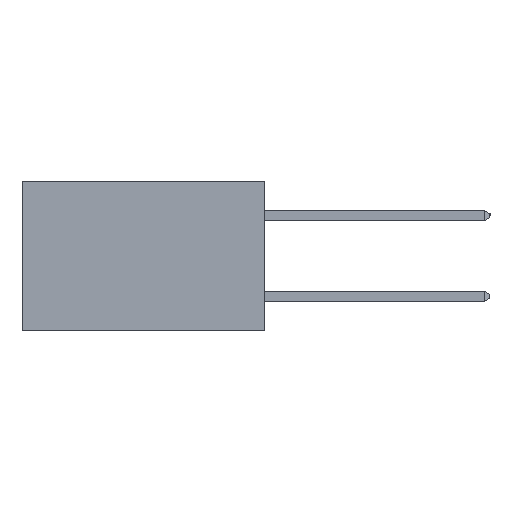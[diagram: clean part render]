
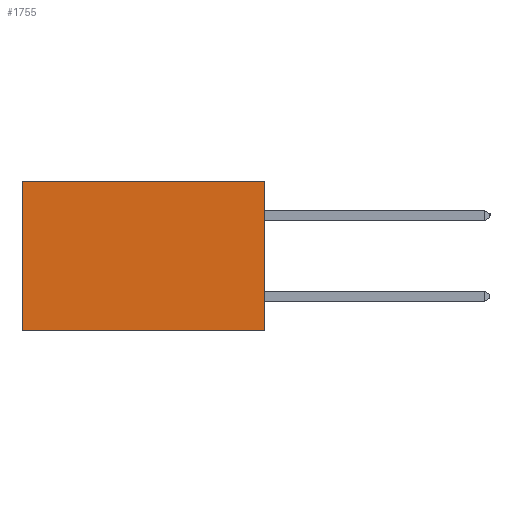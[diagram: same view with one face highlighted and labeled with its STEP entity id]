
A CAD part, left-side view. The second image highlights one B-rep face of the part: STEP entity #1755.
In plain terms, the highlighted planar face has unit normal (-1, 0, 0).
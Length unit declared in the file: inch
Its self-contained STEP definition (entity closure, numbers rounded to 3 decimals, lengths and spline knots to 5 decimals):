
#355 = ORIENTED_EDGE ( 'NONE', *, *, #5531, .T. ) ;
#485 = ORIENTED_EDGE ( 'NONE', *, *, #9100, .F. ) ;
#519 = VERTEX_POINT ( 'NONE', #5094 ) ;
#935 = DIRECTION ( 'NONE',  ( 0., 1., 0. ) ) ;
#1432 = LINE ( 'NONE', #8411, #14731 ) ;
#1681 = LINE ( 'NONE', #14494, #11536 ) ;
#1755 = ADVANCED_FACE ( 'NONE', ( #13725 ), #10812, .F. ) ;
#3118 = ORIENTED_EDGE ( 'NONE', *, *, #9792, .F. ) ;
#3179 = CARTESIAN_POINT ( 'NONE',  ( 0.298, 0., 0. ) ) ;
#3498 = LINE ( 'NONE', #11924, #15955 ) ;
#4749 = EDGE_CURVE ( 'NONE', #14664, #10191, #3498, .T. ) ;
#5094 = CARTESIAN_POINT ( 'NONE',  ( 0.298, 0., -0.37 ) ) ;
#5531 = EDGE_CURVE ( 'NONE', #11937, #14664, #1432, .T. ) ;
#6019 = LINE ( 'NONE', #15826, #15072 ) ;
#7909 = DIRECTION ( 'NONE',  ( 0., 1., 0. ) ) ;
#8411 = CARTESIAN_POINT ( 'NONE',  ( 0.298, 0., 0. ) ) ;
#8684 = DIRECTION ( 'NONE',  ( 0., 0., -1. ) ) ;
#9100 = EDGE_CURVE ( 'NONE', #11937, #519, #1681, .T. ) ;
#9792 = EDGE_CURVE ( 'NONE', #519, #10191, #6019, .T. ) ;
#9852 = CARTESIAN_POINT ( 'NONE',  ( 0.298, 0.6, -0.37 ) ) ;
#10191 = VERTEX_POINT ( 'NONE', #9852 ) ;
#10621 = ORIENTED_EDGE ( 'NONE', *, *, #4749, .T. ) ;
#10795 = CARTESIAN_POINT ( 'NONE',  ( 0.298, 0., 0. ) ) ;
#10812 = PLANE ( 'NONE',  #11677 ) ;
#11536 = VECTOR ( 'NONE', #8684, 39.37008 ) ;
#11677 = AXIS2_PLACEMENT_3D ( 'NONE', #10795, #12424, #12406 ) ;
#11710 = DIRECTION ( 'NONE',  ( 0., 0., -1. ) ) ;
#11924 = CARTESIAN_POINT ( 'NONE',  ( 0.298, 0.6, 0. ) ) ;
#11937 = VERTEX_POINT ( 'NONE', #3179 ) ;
#12406 = DIRECTION ( 'NONE',  ( 0., 0., -1. ) ) ;
#12424 = DIRECTION ( 'NONE',  ( 1., 0., 0. ) ) ;
#13725 = FACE_OUTER_BOUND ( 'NONE', #14390, .T. ) ;
#14390 = EDGE_LOOP ( 'NONE', ( #10621, #3118, #485, #355 ) ) ;
#14494 = CARTESIAN_POINT ( 'NONE',  ( 0.298, 0., 0. ) ) ;
#14664 = VERTEX_POINT ( 'NONE', #15878 ) ;
#14731 = VECTOR ( 'NONE', #7909, 39.37008 ) ;
#15072 = VECTOR ( 'NONE', #935, 39.37008 ) ;
#15826 = CARTESIAN_POINT ( 'NONE',  ( 0.298, 0., -0.37 ) ) ;
#15878 = CARTESIAN_POINT ( 'NONE',  ( 0.298, 0.6, 0. ) ) ;
#15955 = VECTOR ( 'NONE', #11710, 39.37008 ) ;
